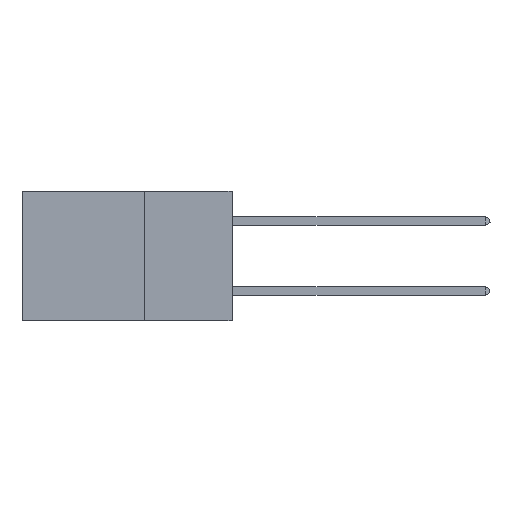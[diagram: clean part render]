
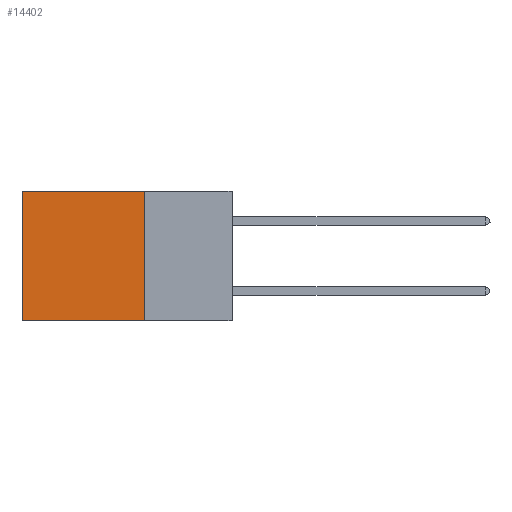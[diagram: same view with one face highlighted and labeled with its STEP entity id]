
A CAD part, left-side view. The second image highlights one B-rep face of the part: STEP entity #14402.
In plain terms, the highlighted planar face has unit normal (-1, 0, 0).
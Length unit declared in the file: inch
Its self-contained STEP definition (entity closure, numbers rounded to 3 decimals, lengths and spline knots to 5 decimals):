
#1678 = EDGE_CURVE ( 'NONE', #4434, #9603, #15639, .T. ) ;
#3407 = LINE ( 'NONE', #19290, #14045 ) ;
#3485 = DIRECTION ( 'NONE',  ( 1., 0., 0. ) ) ;
#4434 = VERTEX_POINT ( 'NONE', #15152 ) ;
#4645 = EDGE_LOOP ( 'NONE', ( #29643, #14201, #14187, #12211 ) ) ;
#4755 = CARTESIAN_POINT ( 'NONE',  ( 0.2875, 0.6, -0.37 ) ) ;
#6431 = CARTESIAN_POINT ( 'NONE',  ( 0.2875, 0.25, -0.37 ) ) ;
#7228 = DIRECTION ( 'NONE',  ( 0., 1., 0. ) ) ;
#9578 = VERTEX_POINT ( 'NONE', #6431 ) ;
#9603 = VERTEX_POINT ( 'NONE', #26375 ) ;
#10298 = FACE_OUTER_BOUND ( 'NONE', #4645, .T. ) ;
#11514 = DIRECTION ( 'NONE',  ( 0., 0., -1. ) ) ;
#12133 = LINE ( 'NONE', #12299, #18099 ) ;
#12211 = ORIENTED_EDGE ( 'NONE', *, *, #1678, .T. ) ;
#12299 = CARTESIAN_POINT ( 'NONE',  ( 0.2875, 0.25, -0.37 ) ) ;
#13161 = LINE ( 'NONE', #17885, #16706 ) ;
#13632 = DIRECTION ( 'NONE',  ( 0., 0., -1. ) ) ;
#13917 = VECTOR ( 'NONE', #26415, 39.37008 ) ;
#14045 = VECTOR ( 'NONE', #11514, 39.37008 ) ;
#14187 = ORIENTED_EDGE ( 'NONE', *, *, #16185, .F. ) ;
#14201 = ORIENTED_EDGE ( 'NONE', *, *, #23454, .F. ) ;
#14402 = ADVANCED_FACE ( 'NONE', ( #10298 ), #24098, .F. ) ;
#15152 = CARTESIAN_POINT ( 'NONE',  ( 0.2875, 0.25, 0. ) ) ;
#15342 = EDGE_CURVE ( 'NONE', #9603, #19913, #3407, .T. ) ;
#15639 = LINE ( 'NONE', #25765, #13917 ) ;
#16185 = EDGE_CURVE ( 'NONE', #4434, #9578, #13161, .T. ) ;
#16339 = CARTESIAN_POINT ( 'NONE',  ( 0.2875, 0.25, 0. ) ) ;
#16706 = VECTOR ( 'NONE', #28197, 39.37008 ) ;
#17885 = CARTESIAN_POINT ( 'NONE',  ( 0.2875, 0.25, 0. ) ) ;
#18099 = VECTOR ( 'NONE', #7228, 39.37008 ) ;
#19290 = CARTESIAN_POINT ( 'NONE',  ( 0.2875, 0.6, 0. ) ) ;
#19913 = VERTEX_POINT ( 'NONE', #4755 ) ;
#23454 = EDGE_CURVE ( 'NONE', #9578, #19913, #12133, .T. ) ;
#24098 = PLANE ( 'NONE',  #32266 ) ;
#25765 = CARTESIAN_POINT ( 'NONE',  ( 0.2875, 0.25, 0. ) ) ;
#26375 = CARTESIAN_POINT ( 'NONE',  ( 0.2875, 0.6, 0. ) ) ;
#26415 = DIRECTION ( 'NONE',  ( 0., 1., 0. ) ) ;
#28197 = DIRECTION ( 'NONE',  ( 0., 0., -1. ) ) ;
#29643 = ORIENTED_EDGE ( 'NONE', *, *, #15342, .T. ) ;
#32266 = AXIS2_PLACEMENT_3D ( 'NONE', #16339, #3485, #13632 ) ;
